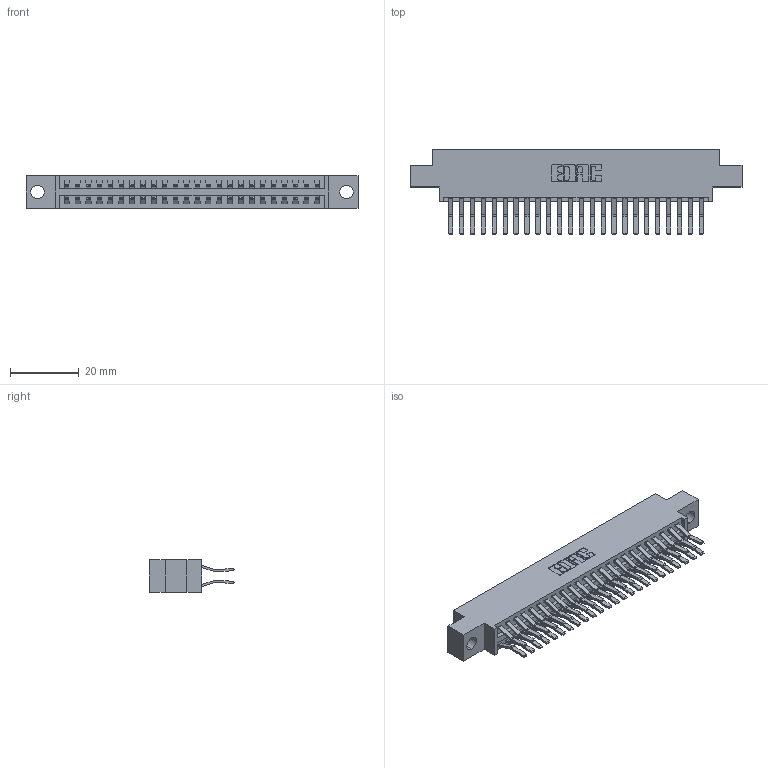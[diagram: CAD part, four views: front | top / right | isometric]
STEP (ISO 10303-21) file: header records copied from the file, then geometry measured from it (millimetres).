
FILE_DESCRIPTION (( 'STEP AP203' ), '1' );
FILE_NAME ('346-048-560-804.STEP', '2022-05-20T22:26:41', ( '' ), ( '' ), 'SwSTEP 2.0', 'SolidWorks 2020', '' );
FILE_SCHEMA (( 'CONFIG_CONTROL_DESIGN' ));
Length unit declared in the file: inch
Products named in the file (3): 345-292-001_560 Tail; 346 Part_0.170 Offset - 0.156 Dia-TH; 346-048-560-804
Assembly tree (49 placements, depth 2):
  346-048-560-804
    346 Part_0.170 Offset - 0.156 Dia-TH
    345-292-001_560 Tail  x48
Bounding box: 96.77 x 24.78 x 9.4 mm (x, y, z)
Volume: 9350.9 mm3; surface area: 13437.5 mm2
Topology: 49 solids, 49 shells, 2732 faces, 8105 edges, 5338 vertices
Faces by surface type: plane 1774, cylinder 958
Entity records: 18725 total; most frequent: CARTESIAN_POINT 3118, ORIENTED_EDGE 3050, DIRECTION 2801, EDGE_CURVE 1525, LINE 1293, VECTOR 1293, VERTEX_POINT 1014, AXIS2_PLACEMENT_3D 754
